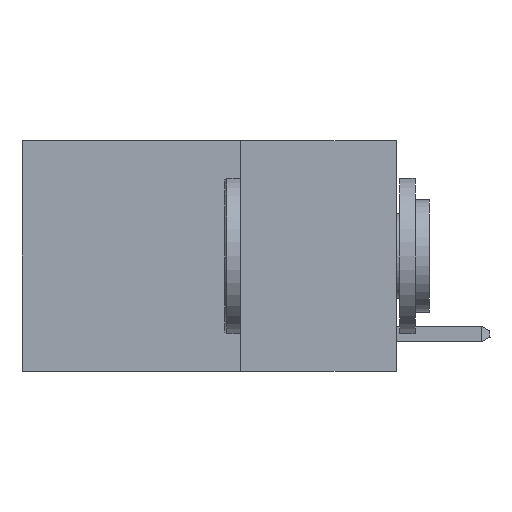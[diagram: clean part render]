
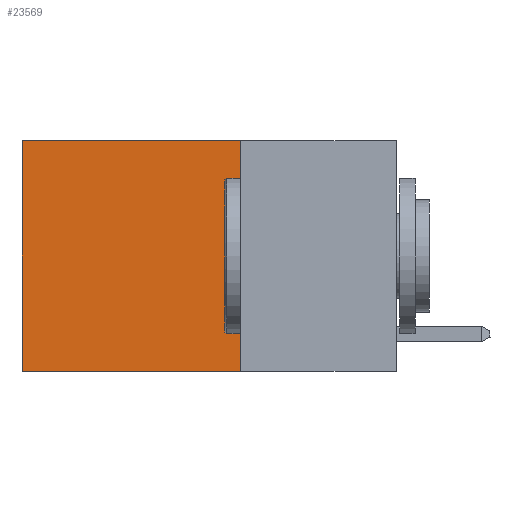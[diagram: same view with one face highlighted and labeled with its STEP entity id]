
A CAD part, left-side view. The second image highlights one B-rep face of the part: STEP entity #23569.
In plain terms, the highlighted planar face has unit normal (-1, 0, 0).
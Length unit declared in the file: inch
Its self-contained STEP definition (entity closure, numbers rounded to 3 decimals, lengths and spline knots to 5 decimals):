
#784 = EDGE_LOOP ( 'NONE', ( #17170, #16492, #22707, #4048 ) ) ;
#1229 = CARTESIAN_POINT ( 'NONE',  ( 0.2625, 0.6, -0.37 ) ) ;
#1602 = VERTEX_POINT ( 'NONE', #2861 ) ;
#1715 = PLANE ( 'NONE',  #15241 ) ;
#2503 = VERTEX_POINT ( 'NONE', #7846 ) ;
#2515 = LINE ( 'NONE', #10334, #20582 ) ;
#2861 = CARTESIAN_POINT ( 'NONE',  ( 0.2625, 0.6, 0. ) ) ;
#4048 = ORIENTED_EDGE ( 'NONE', *, *, #18642, .T. ) ;
#4842 = LINE ( 'NONE', #14785, #7840 ) ;
#6215 = EDGE_CURVE ( 'NONE', #18106, #2503, #10800, .T. ) ;
#6681 = EDGE_CURVE ( 'NONE', #1602, #18819, #7293, .T. ) ;
#7026 = DIRECTION ( 'NONE',  ( 0., 1., 0. ) ) ;
#7293 = LINE ( 'NONE', #15067, #14363 ) ;
#7840 = VECTOR ( 'NONE', #7026, 39.37008 ) ;
#7846 = CARTESIAN_POINT ( 'NONE',  ( 0.2625, 0.25, -0.37 ) ) ;
#9326 = DIRECTION ( 'NONE',  ( 0., 0., -1. ) ) ;
#9520 = CARTESIAN_POINT ( 'NONE',  ( 0.2625, 0.25, 0. ) ) ;
#10334 = CARTESIAN_POINT ( 'NONE',  ( 0.2625, 0.25, 0. ) ) ;
#10800 = LINE ( 'NONE', #22421, #18100 ) ;
#11446 = FACE_OUTER_BOUND ( 'NONE', #784, .T. ) ;
#12713 = DIRECTION ( 'NONE',  ( 0., 0., -1. ) ) ;
#14363 = VECTOR ( 'NONE', #9326, 39.37008 ) ;
#14785 = CARTESIAN_POINT ( 'NONE',  ( 0.2625, 0.25, -0.37 ) ) ;
#14985 = CARTESIAN_POINT ( 'NONE',  ( 0.2625, 0.25, 0. ) ) ;
#15067 = CARTESIAN_POINT ( 'NONE',  ( 0.2625, 0.6, 0. ) ) ;
#15241 = AXIS2_PLACEMENT_3D ( 'NONE', #9520, #19376, #25075 ) ;
#16492 = ORIENTED_EDGE ( 'NONE', *, *, #17025, .F. ) ;
#17025 = EDGE_CURVE ( 'NONE', #2503, #18819, #4842, .T. ) ;
#17170 = ORIENTED_EDGE ( 'NONE', *, *, #6681, .T. ) ;
#18100 = VECTOR ( 'NONE', #12713, 39.37008 ) ;
#18106 = VERTEX_POINT ( 'NONE', #14985 ) ;
#18642 = EDGE_CURVE ( 'NONE', #18106, #1602, #2515, .T. ) ;
#18819 = VERTEX_POINT ( 'NONE', #1229 ) ;
#19376 = DIRECTION ( 'NONE',  ( 1., 0., 0. ) ) ;
#20582 = VECTOR ( 'NONE', #21947, 39.37008 ) ;
#21947 = DIRECTION ( 'NONE',  ( 0., 1., 0. ) ) ;
#22421 = CARTESIAN_POINT ( 'NONE',  ( 0.2625, 0.25, 0. ) ) ;
#22707 = ORIENTED_EDGE ( 'NONE', *, *, #6215, .F. ) ;
#23569 = ADVANCED_FACE ( 'NONE', ( #11446 ), #1715, .F. ) ;
#25075 = DIRECTION ( 'NONE',  ( 0., 0., -1. ) ) ;
